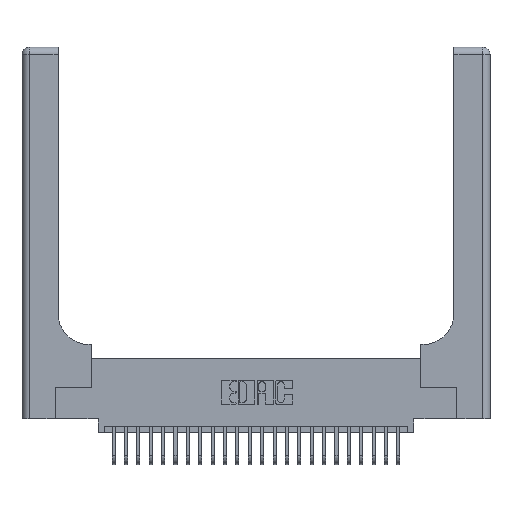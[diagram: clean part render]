
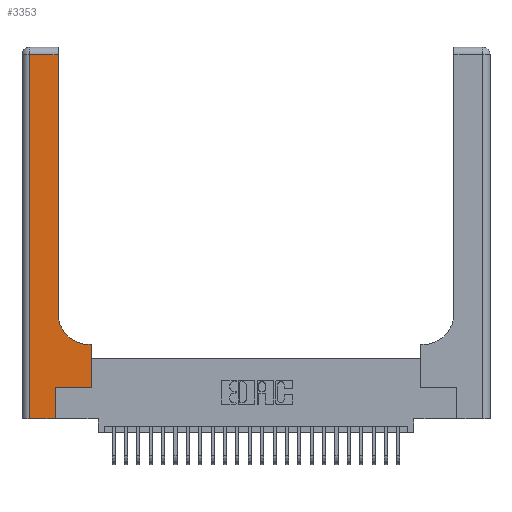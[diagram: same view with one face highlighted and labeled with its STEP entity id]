
A CAD part, top view. The second image highlights one B-rep face of the part: STEP entity #3353.
In plain terms, the highlighted planar face has unit normal (0, 0, 1).
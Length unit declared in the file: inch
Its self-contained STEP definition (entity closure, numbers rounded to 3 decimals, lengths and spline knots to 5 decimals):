
#245 = CARTESIAN_POINT ( 'NONE',  ( 0.5585, 0.25, 0.37 ) ) ;
#304 = CARTESIAN_POINT ( 'NONE',  ( 0.2915, 0.6, 0.37 ) ) ;
#709 = VECTOR ( 'NONE', #13426, 39.37008 ) ;
#1078 = CARTESIAN_POINT ( 'NONE',  ( 0.06, 2.94, 0.37 ) ) ;
#1388 = EDGE_CURVE ( 'NONE', #16927, #7142, #9893, .T. ) ;
#1622 = EDGE_CURVE ( 'NONE', #23149, #15187, #19601, .T. ) ;
#1738 = CIRCLE ( 'NONE', #9378, 0.25 ) ;
#2991 = VECTOR ( 'NONE', #12319, 39.37008 ) ;
#3153 = VERTEX_POINT ( 'NONE', #5662 ) ;
#3353 = ADVANCED_FACE ( 'NONE', ( #10741 ), #8322, .F. ) ;
#3378 = EDGE_CURVE ( 'NONE', #20759, #23149, #10108, .T. ) ;
#3608 = EDGE_CURVE ( 'NONE', #15187, #3153, #1738, .T. ) ;
#5385 = VECTOR ( 'NONE', #16392, 39.37008 ) ;
#5502 = VECTOR ( 'NONE', #9557, 39.37008 ) ;
#5662 = CARTESIAN_POINT ( 'NONE',  ( 0.2915, 0.85, 0.37 ) ) ;
#6316 = LINE ( 'NONE', #9561, #16386 ) ;
#6539 = EDGE_CURVE ( 'NONE', #3153, #14409, #7248, .T. ) ;
#6790 = ORIENTED_EDGE ( 'NONE', *, *, #25547, .T. ) ;
#7142 = VERTEX_POINT ( 'NONE', #16254 ) ;
#7161 = CARTESIAN_POINT ( 'NONE',  ( 0.5415, 0.85, 0.37 ) ) ;
#7248 = LINE ( 'NONE', #13908, #11307 ) ;
#8322 = PLANE ( 'NONE',  #20625 ) ;
#8736 = CARTESIAN_POINT ( 'NONE',  ( 0., 0., 0.37 ) ) ;
#9010 = ORIENTED_EDGE ( 'NONE', *, *, #3378, .T. ) ;
#9168 = DIRECTION ( 'NONE',  ( 1., 0., 0. ) ) ;
#9264 = VECTOR ( 'NONE', #23645, 39.37008 ) ;
#9378 = AXIS2_PLACEMENT_3D ( 'NONE', #7161, #21144, #9168 ) ;
#9557 = DIRECTION ( 'NONE',  ( 0., -1., 0. ) ) ;
#9561 = CARTESIAN_POINT ( 'NONE',  ( 0.269, 0.25, 0.37 ) ) ;
#9671 = CARTESIAN_POINT ( 'NONE',  ( 0.269, 0., 0.37 ) ) ;
#9846 = DIRECTION ( 'NONE',  ( 0., 1., 0. ) ) ;
#9893 = LINE ( 'NONE', #9671, #9264 ) ;
#10108 = LINE ( 'NONE', #245, #5385 ) ;
#10240 = ORIENTED_EDGE ( 'NONE', *, *, #6539, .T. ) ;
#10316 = DIRECTION ( 'NONE',  ( 0., 0., -1. ) ) ;
#10461 = CARTESIAN_POINT ( 'NONE',  ( 0.5585, 0.25, 0.37 ) ) ;
#10741 = FACE_OUTER_BOUND ( 'NONE', #14708, .T. ) ;
#10869 = ORIENTED_EDGE ( 'NONE', *, *, #14900, .T. ) ;
#11307 = VECTOR ( 'NONE', #9846, 39.37008 ) ;
#12265 = CARTESIAN_POINT ( 'NONE',  ( 0., 3., 0.37 ) ) ;
#12273 = CARTESIAN_POINT ( 'NONE',  ( 0.5415, 0.6, 0.37 ) ) ;
#12319 = DIRECTION ( 'NONE',  ( -1., 0., 0. ) ) ;
#13426 = DIRECTION ( 'NONE',  ( -1., 0., 0. ) ) ;
#13516 = CARTESIAN_POINT ( 'NONE',  ( 0., 2.94, 0.37 ) ) ;
#13908 = CARTESIAN_POINT ( 'NONE',  ( 0.2915, 3., 0.37 ) ) ;
#14368 = ORIENTED_EDGE ( 'NONE', *, *, #1622, .T. ) ;
#14409 = VERTEX_POINT ( 'NONE', #25527 ) ;
#14661 = ORIENTED_EDGE ( 'NONE', *, *, #23720, .T. ) ;
#14708 = EDGE_LOOP ( 'NONE', ( #10240, #10869, #6790, #14661, #19961, #23081, #9010, #14368, #16884 ) ) ;
#14900 = EDGE_CURVE ( 'NONE', #14409, #16006, #16735, .T. ) ;
#14943 = LINE ( 'NONE', #19561, #5502 ) ;
#15187 = VERTEX_POINT ( 'NONE', #12273 ) ;
#16006 = VERTEX_POINT ( 'NONE', #1078 ) ;
#16181 = EDGE_CURVE ( 'NONE', #7142, #20759, #6316, .T. ) ;
#16254 = CARTESIAN_POINT ( 'NONE',  ( 0.269, 0.25, 0.37 ) ) ;
#16309 = LINE ( 'NONE', #8736, #20328 ) ;
#16386 = VECTOR ( 'NONE', #25535, 39.37008 ) ;
#16392 = DIRECTION ( 'NONE',  ( 0., 1., 0. ) ) ;
#16646 = CARTESIAN_POINT ( 'NONE',  ( 0.06, 0., 0.37 ) ) ;
#16735 = LINE ( 'NONE', #13516, #709 ) ;
#16884 = ORIENTED_EDGE ( 'NONE', *, *, #3608, .T. ) ;
#16927 = VERTEX_POINT ( 'NONE', #23765 ) ;
#18441 = VERTEX_POINT ( 'NONE', #16646 ) ;
#19561 = CARTESIAN_POINT ( 'NONE',  ( 0.06, 3., 0.37 ) ) ;
#19601 = LINE ( 'NONE', #304, #2991 ) ;
#19961 = ORIENTED_EDGE ( 'NONE', *, *, #1388, .T. ) ;
#20328 = VECTOR ( 'NONE', #24616, 39.37008 ) ;
#20625 = AXIS2_PLACEMENT_3D ( 'NONE', #12265, #10316, #24268 ) ;
#20759 = VERTEX_POINT ( 'NONE', #10461 ) ;
#21144 = DIRECTION ( 'NONE',  ( 0., 0., -1. ) ) ;
#23081 = ORIENTED_EDGE ( 'NONE', *, *, #16181, .T. ) ;
#23149 = VERTEX_POINT ( 'NONE', #24823 ) ;
#23645 = DIRECTION ( 'NONE',  ( 0., 1., 0. ) ) ;
#23720 = EDGE_CURVE ( 'NONE', #18441, #16927, #16309, .T. ) ;
#23765 = CARTESIAN_POINT ( 'NONE',  ( 0.269, 0., 0.37 ) ) ;
#24268 = DIRECTION ( 'NONE',  ( -1., 0., 0. ) ) ;
#24616 = DIRECTION ( 'NONE',  ( 1., 0., 0. ) ) ;
#24823 = CARTESIAN_POINT ( 'NONE',  ( 0.5585, 0.6, 0.37 ) ) ;
#25527 = CARTESIAN_POINT ( 'NONE',  ( 0.2915, 2.94, 0.37 ) ) ;
#25535 = DIRECTION ( 'NONE',  ( 1., 0., 0. ) ) ;
#25547 = EDGE_CURVE ( 'NONE', #16006, #18441, #14943, .T. ) ;
